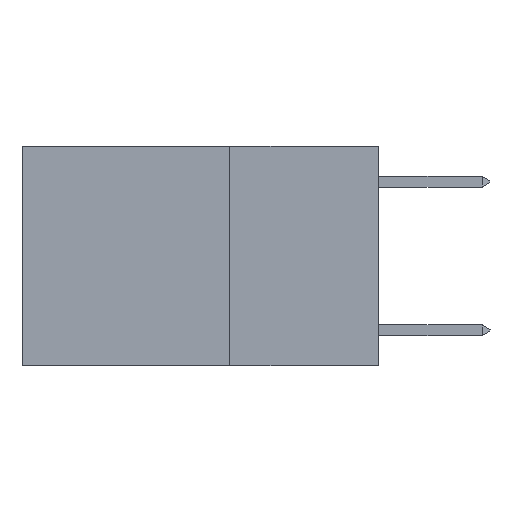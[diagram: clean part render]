
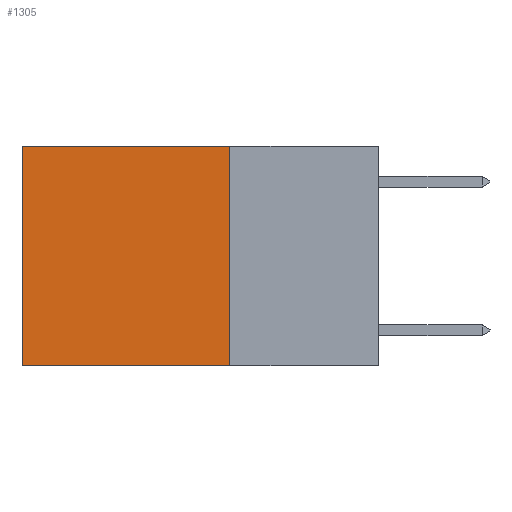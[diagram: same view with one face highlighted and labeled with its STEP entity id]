
A CAD part, left-side view. The second image highlights one B-rep face of the part: STEP entity #1305.
In plain terms, the highlighted planar face has unit normal (-1, 0, 0).
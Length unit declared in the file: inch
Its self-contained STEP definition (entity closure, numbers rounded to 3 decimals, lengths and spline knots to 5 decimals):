
#884 = DIRECTION ( 'NONE',  ( 0., 0., -1. ) ) ;
#1305 = ADVANCED_FACE ( 'NONE', ( #6089 ), #10820, .F. ) ;
#1434 = EDGE_LOOP ( 'NONE', ( #5674, #2027, #13138, #2473 ) ) ;
#2027 = ORIENTED_EDGE ( 'NONE', *, *, #9353, .F. ) ;
#2414 = EDGE_CURVE ( 'NONE', #6908, #5565, #6547, .T. ) ;
#2473 = ORIENTED_EDGE ( 'NONE', *, *, #7772, .T. ) ;
#3584 = AXIS2_PLACEMENT_3D ( 'NONE', #4553, #11881, #5648 ) ;
#4025 = CARTESIAN_POINT ( 'NONE',  ( 0.2625, 0.6, 0. ) ) ;
#4553 = CARTESIAN_POINT ( 'NONE',  ( 0.2625, 0.25, 0. ) ) ;
#4744 = VECTOR ( 'NONE', #5105, 39.37008 ) ;
#5099 = LINE ( 'NONE', #7544, #7908 ) ;
#5105 = DIRECTION ( 'NONE',  ( 0., 0., -1. ) ) ;
#5404 = VECTOR ( 'NONE', #9333, 39.37008 ) ;
#5565 = VERTEX_POINT ( 'NONE', #5742 ) ;
#5648 = DIRECTION ( 'NONE',  ( 0., 0., -1. ) ) ;
#5674 = ORIENTED_EDGE ( 'NONE', *, *, #9331, .T. ) ;
#5742 = CARTESIAN_POINT ( 'NONE',  ( 0.2625, 0.25, -0.37 ) ) ;
#6089 = FACE_OUTER_BOUND ( 'NONE', #1434, .T. ) ;
#6547 = LINE ( 'NONE', #8708, #11733 ) ;
#6908 = VERTEX_POINT ( 'NONE', #12438 ) ;
#6958 = VERTEX_POINT ( 'NONE', #9378 ) ;
#7122 = CARTESIAN_POINT ( 'NONE',  ( 0.2625, 0.6, -0.37 ) ) ;
#7544 = CARTESIAN_POINT ( 'NONE',  ( 0.2625, 0.25, 0. ) ) ;
#7550 = LINE ( 'NONE', #8288, #5404 ) ;
#7772 = EDGE_CURVE ( 'NONE', #6908, #6958, #5099, .T. ) ;
#7908 = VECTOR ( 'NONE', #8591, 39.37008 ) ;
#8288 = CARTESIAN_POINT ( 'NONE',  ( 0.2625, 0.25, -0.37 ) ) ;
#8591 = DIRECTION ( 'NONE',  ( 0., 1., 0. ) ) ;
#8708 = CARTESIAN_POINT ( 'NONE',  ( 0.2625, 0.25, 0. ) ) ;
#9331 = EDGE_CURVE ( 'NONE', #6958, #13612, #13070, .T. ) ;
#9333 = DIRECTION ( 'NONE',  ( 0., 1., 0. ) ) ;
#9353 = EDGE_CURVE ( 'NONE', #5565, #13612, #7550, .T. ) ;
#9378 = CARTESIAN_POINT ( 'NONE',  ( 0.2625, 0.6, 0. ) ) ;
#10820 = PLANE ( 'NONE',  #3584 ) ;
#11733 = VECTOR ( 'NONE', #884, 39.37008 ) ;
#11881 = DIRECTION ( 'NONE',  ( 1., 0., 0. ) ) ;
#12438 = CARTESIAN_POINT ( 'NONE',  ( 0.2625, 0.25, 0. ) ) ;
#13070 = LINE ( 'NONE', #4025, #4744 ) ;
#13138 = ORIENTED_EDGE ( 'NONE', *, *, #2414, .F. ) ;
#13612 = VERTEX_POINT ( 'NONE', #7122 ) ;
